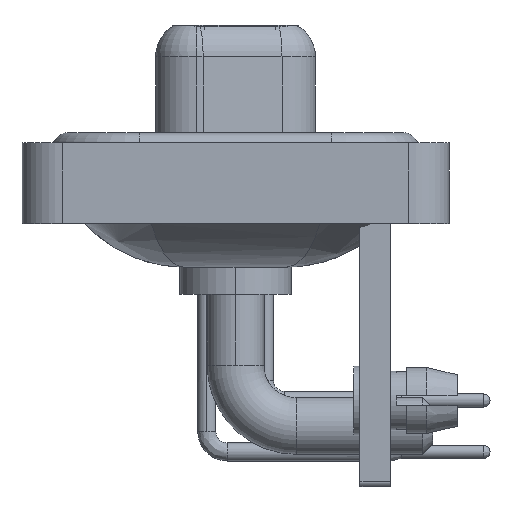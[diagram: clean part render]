
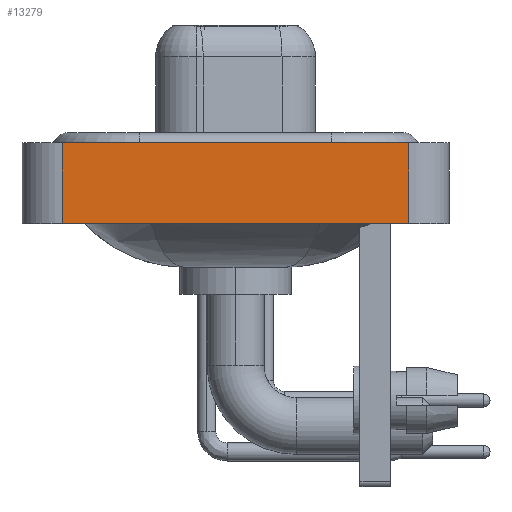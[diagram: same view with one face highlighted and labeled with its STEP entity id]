
A CAD part, left-side view. The second image highlights one B-rep face of the part: STEP entity #13279.
In plain terms, the highlighted planar face has unit normal (-1, 0, 0).
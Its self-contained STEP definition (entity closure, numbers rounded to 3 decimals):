
#423 = DIRECTION ( 'NONE',  ( 0., -1., 0. ) ) ;
#897 = VERTEX_POINT ( 'NONE', #11489 ) ;
#1298 = LINE ( 'NONE', #20720, #5349 ) ;
#1594 = DIRECTION ( 'NONE',  ( 0., -1., 0. ) ) ;
#1602 = LINE ( 'NONE', #19641, #12349 ) ;
#2578 = ORIENTED_EDGE ( 'NONE', *, *, #17858, .T. ) ;
#3501 = EDGE_CURVE ( 'NONE', #3678, #12279, #22047, .T. ) ;
#3673 = VECTOR ( 'NONE', #423, 1000. ) ;
#3678 = VERTEX_POINT ( 'NONE', #15267 ) ;
#3845 = CARTESIAN_POINT ( 'NONE',  ( -7.3, -8.55, 0.4 ) ) ;
#5078 = EDGE_CURVE ( 'NONE', #20769, #897, #19272, .T. ) ;
#5349 = VECTOR ( 'NONE', #11892, 1000. ) ;
#6541 = EDGE_LOOP ( 'NONE', ( #2578, #9423, #18494, #16898 ) ) ;
#6599 = CARTESIAN_POINT ( 'NONE',  ( -7.3, -8.55, -3.6 ) ) ;
#7343 = AXIS2_PLACEMENT_3D ( 'NONE', #8254, #22244, #15345 ) ;
#8254 = CARTESIAN_POINT ( 'NONE',  ( -7.3, -8.55, -3.6 ) ) ;
#8292 = VECTOR ( 'NONE', #1594, 1000. ) ;
#9423 = ORIENTED_EDGE ( 'NONE', *, *, #3501, .F. ) ;
#11489 = CARTESIAN_POINT ( 'NONE',  ( -7.3, -8.55, -3.6 ) ) ;
#11892 = DIRECTION ( 'NONE',  ( 0., 0., 1. ) ) ;
#12279 = VERTEX_POINT ( 'NONE', #3845 ) ;
#12349 = VECTOR ( 'NONE', #22910, 1000. ) ;
#13279 = ADVANCED_FACE ( 'NONE', ( #18498 ), #18728, .T. ) ;
#14913 = CARTESIAN_POINT ( 'NONE',  ( -7.3, -8.55, 0.4 ) ) ;
#15267 = CARTESIAN_POINT ( 'NONE',  ( -7.3, 8.55, 0.4 ) ) ;
#15345 = DIRECTION ( 'NONE',  ( 0., 0., 1. ) ) ;
#15555 = EDGE_CURVE ( 'NONE', #20769, #3678, #1298, .T. ) ;
#16898 = ORIENTED_EDGE ( 'NONE', *, *, #5078, .T. ) ;
#17858 = EDGE_CURVE ( 'NONE', #897, #12279, #1602, .T. ) ;
#18494 = ORIENTED_EDGE ( 'NONE', *, *, #15555, .F. ) ;
#18498 = FACE_OUTER_BOUND ( 'NONE', #6541, .T. ) ;
#18728 = PLANE ( 'NONE',  #7343 ) ;
#19272 = LINE ( 'NONE', #6599, #8292 ) ;
#19641 = CARTESIAN_POINT ( 'NONE',  ( -7.3, -8.55, -3.6 ) ) ;
#20720 = CARTESIAN_POINT ( 'NONE',  ( -7.3, 8.55, -3.6 ) ) ;
#20769 = VERTEX_POINT ( 'NONE', #21673 ) ;
#21673 = CARTESIAN_POINT ( 'NONE',  ( -7.3, 8.55, -3.6 ) ) ;
#22047 = LINE ( 'NONE', #14913, #3673 ) ;
#22244 = DIRECTION ( 'NONE',  ( -1., 0., 0. ) ) ;
#22910 = DIRECTION ( 'NONE',  ( 0., 0., 1. ) ) ;
